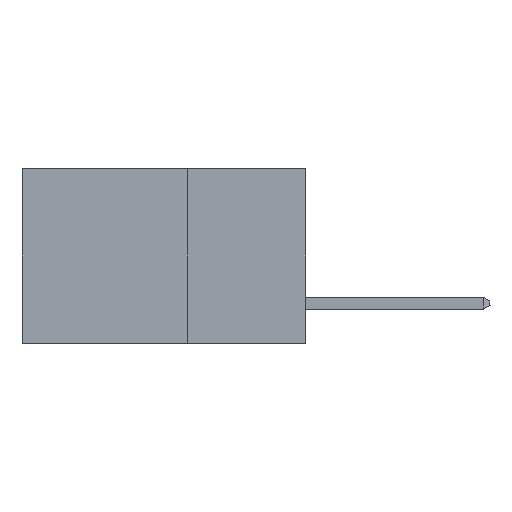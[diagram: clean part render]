
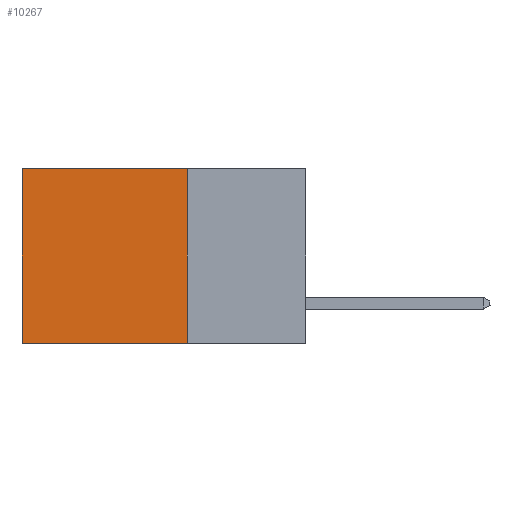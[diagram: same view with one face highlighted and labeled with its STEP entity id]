
A CAD part, left-side view. The second image highlights one B-rep face of the part: STEP entity #10267.
In plain terms, the highlighted planar face has unit normal (-1, 0, 0).
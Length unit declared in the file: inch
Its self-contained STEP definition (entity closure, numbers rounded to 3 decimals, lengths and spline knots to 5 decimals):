
#212 = CARTESIAN_POINT ( 'NONE',  ( 0.298, 0.25, 0. ) ) ;
#912 = EDGE_CURVE ( 'NONE', #9622, #4095, #7446, .T. ) ;
#1340 = VECTOR ( 'NONE', #10364, 39.37008 ) ;
#1381 = ORIENTED_EDGE ( 'NONE', *, *, #912, .T. ) ;
#1657 = EDGE_CURVE ( 'NONE', #8244, #3088, #4631, .T. ) ;
#1723 = AXIS2_PLACEMENT_3D ( 'NONE', #6873, #4023, #6827 ) ;
#2223 = CARTESIAN_POINT ( 'NONE',  ( 0.298, 0.6, 0. ) ) ;
#3088 = VERTEX_POINT ( 'NONE', #3774 ) ;
#3209 = VECTOR ( 'NONE', #6757, 39.37008 ) ;
#3581 = DIRECTION ( 'NONE',  ( 0., 0., -1. ) ) ;
#3743 = EDGE_CURVE ( 'NONE', #8244, #9622, #10583, .T. ) ;
#3774 = CARTESIAN_POINT ( 'NONE',  ( 0.298, 0.25, -0.37 ) ) ;
#3973 = EDGE_CURVE ( 'NONE', #3088, #4095, #5045, .T. ) ;
#4023 = DIRECTION ( 'NONE',  ( 1., 0., 0. ) ) ;
#4095 = VERTEX_POINT ( 'NONE', #5030 ) ;
#4631 = LINE ( 'NONE', #212, #8927 ) ;
#4763 = ORIENTED_EDGE ( 'NONE', *, *, #3743, .T. ) ;
#4809 = VECTOR ( 'NONE', #3581, 39.37008 ) ;
#5030 = CARTESIAN_POINT ( 'NONE',  ( 0.298, 0.6, -0.37 ) ) ;
#5045 = LINE ( 'NONE', #10773, #3209 ) ;
#6757 = DIRECTION ( 'NONE',  ( 0., 1., 0. ) ) ;
#6827 = DIRECTION ( 'NONE',  ( 0., 0., -1. ) ) ;
#6873 = CARTESIAN_POINT ( 'NONE',  ( 0.298, 0.25, 0. ) ) ;
#7027 = ORIENTED_EDGE ( 'NONE', *, *, #3973, .F. ) ;
#7446 = LINE ( 'NONE', #2223, #4809 ) ;
#8244 = VERTEX_POINT ( 'NONE', #8949 ) ;
#8927 = VECTOR ( 'NONE', #11914, 39.37008 ) ;
#8949 = CARTESIAN_POINT ( 'NONE',  ( 0.298, 0.25, 0. ) ) ;
#9622 = VERTEX_POINT ( 'NONE', #12012 ) ;
#9759 = ORIENTED_EDGE ( 'NONE', *, *, #1657, .F. ) ;
#9787 = PLANE ( 'NONE',  #1723 ) ;
#10267 = ADVANCED_FACE ( 'NONE', ( #10329 ), #9787, .F. ) ;
#10329 = FACE_OUTER_BOUND ( 'NONE', #12157, .T. ) ;
#10364 = DIRECTION ( 'NONE',  ( 0., 1., 0. ) ) ;
#10583 = LINE ( 'NONE', #11344, #1340 ) ;
#10773 = CARTESIAN_POINT ( 'NONE',  ( 0.298, 0.25, -0.37 ) ) ;
#11344 = CARTESIAN_POINT ( 'NONE',  ( 0.298, 0.25, 0. ) ) ;
#11914 = DIRECTION ( 'NONE',  ( 0., 0., -1. ) ) ;
#12012 = CARTESIAN_POINT ( 'NONE',  ( 0.298, 0.6, 0. ) ) ;
#12157 = EDGE_LOOP ( 'NONE', ( #1381, #7027, #9759, #4763 ) ) ;
